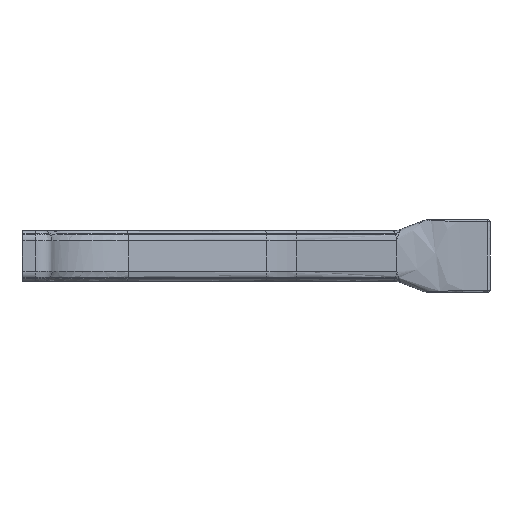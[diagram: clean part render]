
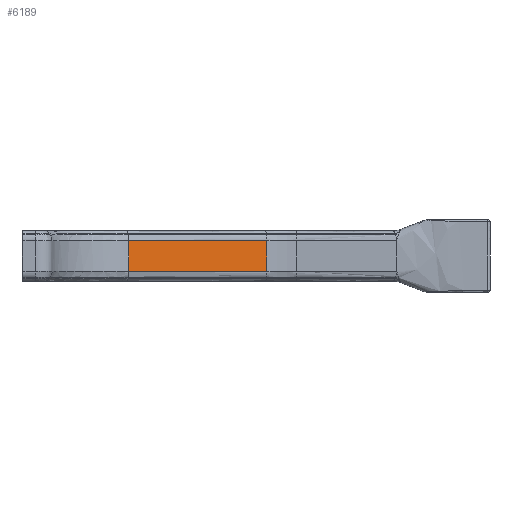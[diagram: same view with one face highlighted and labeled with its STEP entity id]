
A CAD part, front view. The second image highlights one B-rep face of the part: STEP entity #6189.
In plain terms, the highlighted planar face has unit normal (0.186, -0.983, 0).
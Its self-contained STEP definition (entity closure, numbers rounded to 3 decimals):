
#1056 = VECTOR ( 'NONE', #12813, 1000. ) ;
#1800 = ORIENTED_EDGE ( 'NONE', *, *, #10031, .F. ) ;
#2722 = AXIS2_PLACEMENT_3D ( 'NONE', #12806, #10622, #14140 ) ;
#2740 = EDGE_CURVE ( 'NONE', #13417, #14958, #10455, .T. ) ;
#3034 = CARTESIAN_POINT ( 'NONE',  ( -352.416, -4.508, 7.341 ) ) ;
#3226 = EDGE_CURVE ( 'NONE', #10226, #5614, #8834, .T. ) ;
#3698 = CARTESIAN_POINT ( 'NONE',  ( -410.661, -15.544, -7.895 ) ) ;
#4500 = VECTOR ( 'NONE', #12478, 1000. ) ;
#4868 = LINE ( 'NONE', #3034, #4500 ) ;
#4878 = DIRECTION ( 'NONE',  ( 0., 0., -1. ) ) ;
#5365 = CARTESIAN_POINT ( 'NONE',  ( -342.396, -2.61, 7.341 ) ) ;
#5460 = FACE_OUTER_BOUND ( 'NONE', #7579, .T. ) ;
#5591 = DIRECTION ( 'NONE',  ( -0.983, -0.186, 0. ) ) ;
#5614 = VERTEX_POINT ( 'NONE', #6553 ) ;
#5806 = VECTOR ( 'NONE', #5591, 1000. ) ;
#6189 = ADVANCED_FACE ( 'NONE', ( #5460 ), #10409, .T. ) ;
#6553 = CARTESIAN_POINT ( 'NONE',  ( -410.661, -15.544, -7.895 ) ) ;
#7579 = EDGE_LOOP ( 'NONE', ( #1800, #10259, #9733, #15110 ) ) ;
#7747 = CARTESIAN_POINT ( 'NONE',  ( -342.396, -2.61, -7.895 ) ) ;
#8152 = CARTESIAN_POINT ( 'NONE',  ( -410.661, -15.544, 7.341 ) ) ;
#8646 = VECTOR ( 'NONE', #4878, 1000. ) ;
#8834 = LINE ( 'NONE', #3698, #8646 ) ;
#9492 = CARTESIAN_POINT ( 'NONE',  ( -342.396, -2.61, -15.838 ) ) ;
#9733 = ORIENTED_EDGE ( 'NONE', *, *, #11325, .F. ) ;
#10031 = EDGE_CURVE ( 'NONE', #10226, #13417, #4868, .T. ) ;
#10226 = VERTEX_POINT ( 'NONE', #8152 ) ;
#10259 = ORIENTED_EDGE ( 'NONE', *, *, #3226, .T. ) ;
#10409 = PLANE ( 'NONE',  #2722 ) ;
#10455 = LINE ( 'NONE', #9492, #1056 ) ;
#10622 = DIRECTION ( 'NONE',  ( 0.186, -0.983, 0. ) ) ;
#11325 = EDGE_CURVE ( 'NONE', #14958, #5614, #14448, .T. ) ;
#11423 = CARTESIAN_POINT ( 'NONE',  ( -352.416, -4.508, -7.895 ) ) ;
#12478 = DIRECTION ( 'NONE',  ( 0.983, 0.186, 0. ) ) ;
#12806 = CARTESIAN_POINT ( 'NONE',  ( -345.02, -3.107, -15.838 ) ) ;
#12813 = DIRECTION ( 'NONE',  ( 0., 0., -1. ) ) ;
#13417 = VERTEX_POINT ( 'NONE', #5365 ) ;
#14140 = DIRECTION ( 'NONE',  ( 0., 0., 1. ) ) ;
#14448 = LINE ( 'NONE', #11423, #5806 ) ;
#14958 = VERTEX_POINT ( 'NONE', #7747 ) ;
#15110 = ORIENTED_EDGE ( 'NONE', *, *, #2740, .F. ) ;
